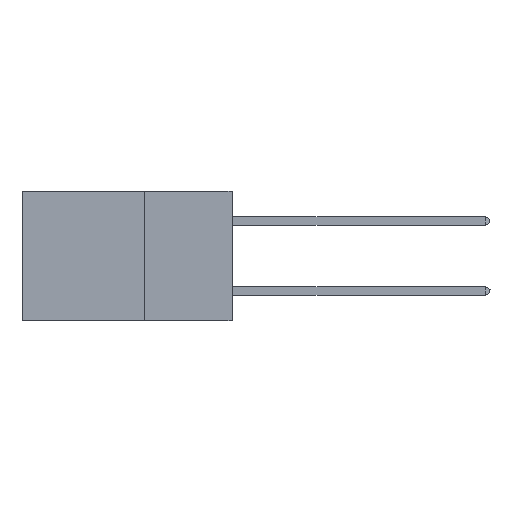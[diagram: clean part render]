
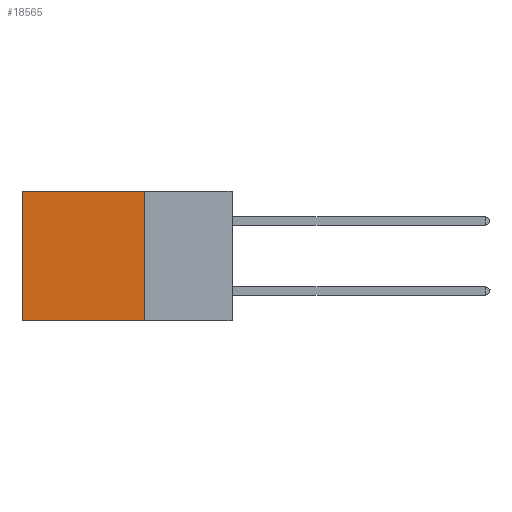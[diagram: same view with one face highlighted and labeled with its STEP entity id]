
A CAD part, left-side view. The second image highlights one B-rep face of the part: STEP entity #18565.
In plain terms, the highlighted planar face has unit normal (-1, 0, 0).
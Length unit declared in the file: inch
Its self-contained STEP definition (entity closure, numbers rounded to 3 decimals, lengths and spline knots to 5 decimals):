
#1462 = ORIENTED_EDGE ( 'NONE', *, *, #31270, .T. ) ;
#4223 = DIRECTION ( 'NONE',  ( 1., 0., 0. ) ) ;
#4600 = EDGE_CURVE ( 'NONE', #10754, #37818, #39393, .T. ) ;
#4802 = CARTESIAN_POINT ( 'NONE',  ( 0.2875, 0.25, -0.37 ) ) ;
#6845 = CARTESIAN_POINT ( 'NONE',  ( 0.2875, 0.6, 0. ) ) ;
#7134 = CARTESIAN_POINT ( 'NONE',  ( 0.2875, 0.25, 0. ) ) ;
#7849 = LINE ( 'NONE', #23276, #21586 ) ;
#8314 = CARTESIAN_POINT ( 'NONE',  ( 0.2875, 0.6, -0.37 ) ) ;
#9370 = LINE ( 'NONE', #6845, #18195 ) ;
#10016 = DIRECTION ( 'NONE',  ( 0., 0., -1. ) ) ;
#10754 = VERTEX_POINT ( 'NONE', #42123 ) ;
#13707 = DIRECTION ( 'NONE',  ( 0., 1., 0. ) ) ;
#14619 = CARTESIAN_POINT ( 'NONE',  ( 0.2875, 0.6, 0. ) ) ;
#15412 = EDGE_CURVE ( 'NONE', #42159, #10754, #30433, .T. ) ;
#15918 = ORIENTED_EDGE ( 'NONE', *, *, #38141, .T. ) ;
#15993 = ORIENTED_EDGE ( 'NONE', *, *, #15412, .F. ) ;
#17521 = DIRECTION ( 'NONE',  ( 0., 0., -1. ) ) ;
#18195 = VECTOR ( 'NONE', #37110, 39.37008 ) ;
#18565 = ADVANCED_FACE ( 'NONE', ( #34353 ), #24437, .F. ) ;
#20828 = VECTOR ( 'NONE', #24876, 39.37008 ) ;
#21586 = VECTOR ( 'NONE', #13707, 39.37008 ) ;
#23276 = CARTESIAN_POINT ( 'NONE',  ( 0.2875, 0.25, 0. ) ) ;
#23816 = VERTEX_POINT ( 'NONE', #14619 ) ;
#24437 = PLANE ( 'NONE',  #37312 ) ;
#24876 = DIRECTION ( 'NONE',  ( 0., 1., 0. ) ) ;
#26907 = CARTESIAN_POINT ( 'NONE',  ( 0.2875, 0.25, 0. ) ) ;
#30433 = LINE ( 'NONE', #7134, #41230 ) ;
#31270 = EDGE_CURVE ( 'NONE', #42159, #23816, #7849, .T. ) ;
#31747 = ORIENTED_EDGE ( 'NONE', *, *, #4600, .F. ) ;
#33702 = CARTESIAN_POINT ( 'NONE',  ( 0.2875, 0.25, 0. ) ) ;
#34353 = FACE_OUTER_BOUND ( 'NONE', #42648, .T. ) ;
#37110 = DIRECTION ( 'NONE',  ( 0., 0., -1. ) ) ;
#37312 = AXIS2_PLACEMENT_3D ( 'NONE', #33702, #4223, #17521 ) ;
#37818 = VERTEX_POINT ( 'NONE', #8314 ) ;
#38141 = EDGE_CURVE ( 'NONE', #23816, #37818, #9370, .T. ) ;
#39393 = LINE ( 'NONE', #4802, #20828 ) ;
#41230 = VECTOR ( 'NONE', #10016, 39.37008 ) ;
#42123 = CARTESIAN_POINT ( 'NONE',  ( 0.2875, 0.25, -0.37 ) ) ;
#42159 = VERTEX_POINT ( 'NONE', #26907 ) ;
#42648 = EDGE_LOOP ( 'NONE', ( #15918, #31747, #15993, #1462 ) ) ;
